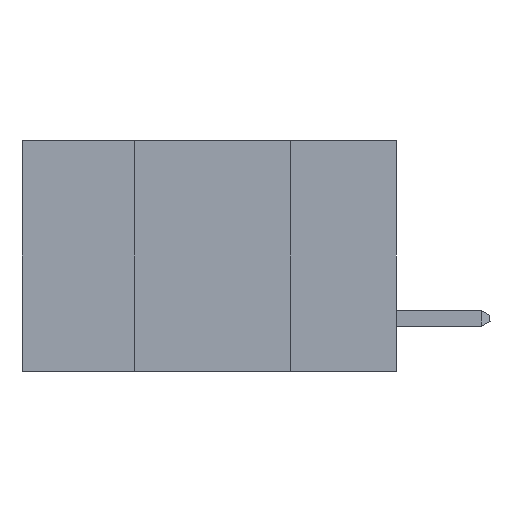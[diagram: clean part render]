
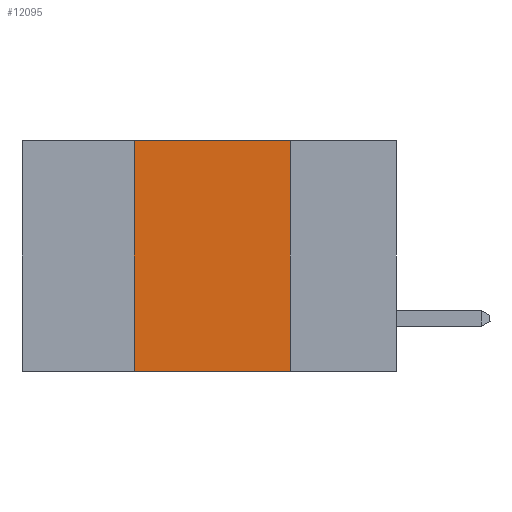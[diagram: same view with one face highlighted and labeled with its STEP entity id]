
A CAD part, left-side view. The second image highlights one B-rep face of the part: STEP entity #12095.
In plain terms, the highlighted planar face has unit normal (-1, 0, 0).
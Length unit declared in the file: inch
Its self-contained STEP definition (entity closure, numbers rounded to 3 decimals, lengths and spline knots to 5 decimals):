
#1375 = ORIENTED_EDGE ( 'NONE', *, *, #18717, .T. ) ;
#1543 = VERTEX_POINT ( 'NONE', #16211 ) ;
#1791 = PLANE ( 'NONE',  #16976 ) ;
#1855 = DIRECTION ( 'NONE',  ( 0., -1., 0. ) ) ;
#2101 = CARTESIAN_POINT ( 'NONE',  ( 0., 0.6, 0. ) ) ;
#2429 = EDGE_LOOP ( 'NONE', ( #11344, #7077, #16989, #1375 ) ) ;
#3568 = DIRECTION ( 'NONE',  ( 0., 0., -1. ) ) ;
#4291 = LINE ( 'NONE', #2101, #12822 ) ;
#4675 = CARTESIAN_POINT ( 'NONE',  ( 0., 0.42, 0. ) ) ;
#5205 = CARTESIAN_POINT ( 'NONE',  ( 0., 0.17, 0. ) ) ;
#5218 = VERTEX_POINT ( 'NONE', #13765 ) ;
#6172 = VECTOR ( 'NONE', #15180, 39.37008 ) ;
#7072 = CARTESIAN_POINT ( 'NONE',  ( 0., 0.6, -0.37 ) ) ;
#7077 = ORIENTED_EDGE ( 'NONE', *, *, #10284, .F. ) ;
#8806 = CARTESIAN_POINT ( 'NONE',  ( 0., 0.42, -0.37 ) ) ;
#9178 = VERTEX_POINT ( 'NONE', #5205 ) ;
#10284 = EDGE_CURVE ( 'NONE', #5218, #9178, #4291, .T. ) ;
#10377 = CARTESIAN_POINT ( 'NONE',  ( 0., 0.6, 0. ) ) ;
#10416 = EDGE_CURVE ( 'NONE', #9178, #1543, #15258, .T. ) ;
#11344 = ORIENTED_EDGE ( 'NONE', *, *, #10416, .F. ) ;
#12095 = ADVANCED_FACE ( 'NONE', ( #20858 ), #1791, .F. ) ;
#12476 = LINE ( 'NONE', #7072, #21018 ) ;
#12822 = VECTOR ( 'NONE', #1855, 39.37008 ) ;
#13485 = VERTEX_POINT ( 'NONE', #8806 ) ;
#13765 = CARTESIAN_POINT ( 'NONE',  ( 0., 0.42, 0. ) ) ;
#13823 = DIRECTION ( 'NONE',  ( 1., 0., 0. ) ) ;
#14875 = LINE ( 'NONE', #4675, #19943 ) ;
#15180 = DIRECTION ( 'NONE',  ( 0., 0., -1. ) ) ;
#15258 = LINE ( 'NONE', #15412, #6172 ) ;
#15412 = CARTESIAN_POINT ( 'NONE',  ( 0., 0.17, 0. ) ) ;
#15449 = EDGE_CURVE ( 'NONE', #13485, #5218, #14875, .T. ) ;
#15660 = DIRECTION ( 'NONE',  ( 0., -1., 0. ) ) ;
#16211 = CARTESIAN_POINT ( 'NONE',  ( 0., 0.17, -0.37 ) ) ;
#16976 = AXIS2_PLACEMENT_3D ( 'NONE', #10377, #13823, #3568 ) ;
#16989 = ORIENTED_EDGE ( 'NONE', *, *, #15449, .F. ) ;
#18373 = DIRECTION ( 'NONE',  ( 0., 0., 1. ) ) ;
#18717 = EDGE_CURVE ( 'NONE', #13485, #1543, #12476, .T. ) ;
#19943 = VECTOR ( 'NONE', #18373, 39.37008 ) ;
#20858 = FACE_OUTER_BOUND ( 'NONE', #2429, .T. ) ;
#21018 = VECTOR ( 'NONE', #15660, 39.37008 ) ;
